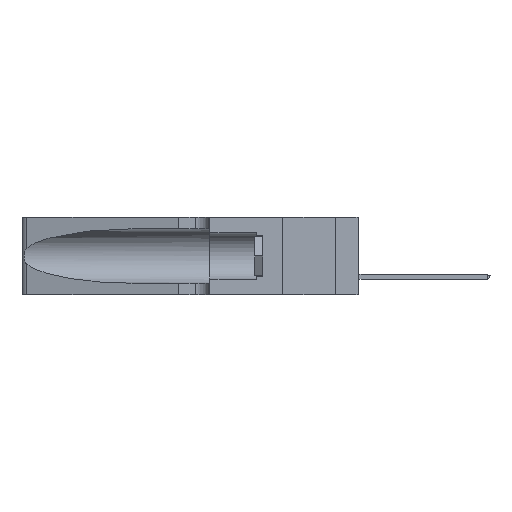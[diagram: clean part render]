
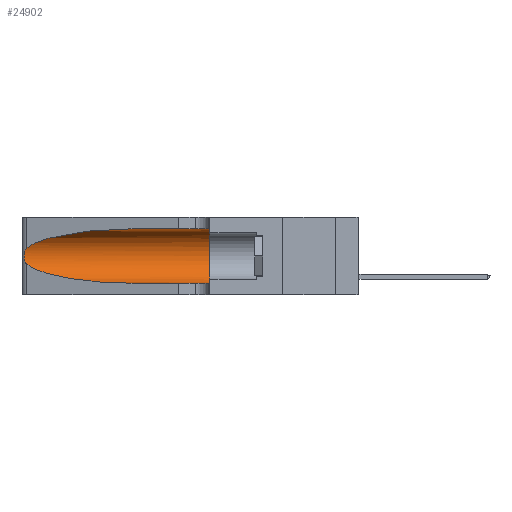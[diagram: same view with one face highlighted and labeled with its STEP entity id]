
A CAD part, left-side view. The second image highlights one B-rep face of the part: STEP entity #24902.
In plain terms, the highlighted cylindrical face has radius 3.308 mm (diameter 6.617 mm), a partial arc.
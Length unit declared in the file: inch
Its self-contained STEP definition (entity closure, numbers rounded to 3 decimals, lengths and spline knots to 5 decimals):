
#1590 = CARTESIAN_POINT ( 'NONE',  ( 0.1305, 0.35, 0.31525 ) ) ;
#2297 = CYLINDRICAL_SURFACE ( 'NONE', #27522, 0.13025 ) ;
#3438 = FACE_OUTER_BOUND ( 'NONE', #16273, .T. ) ;
#4509 = CARTESIAN_POINT ( 'NONE',  ( 0.25487, 1.22718, 0.14631 ) ) ;
#4609 = EDGE_CURVE ( 'NONE', #43980, #24915, #43379, .T. ) ;
#4656 = LINE ( 'NONE', #34526, #8044 ) ;
#4694 = AXIS2_PLACEMENT_3D ( 'NONE', #8359, #11439, #29441 ) ;
#4831 = CARTESIAN_POINT ( 'NONE',  ( 0.18966, 0.96281, 0.05475 ) ) ;
#5247 = CARTESIAN_POINT ( 'NONE',  ( 0.25487, 1.22718, 0.14631 ) ) ;
#6354 = VERTEX_POINT ( 'NONE', #29398 ) ;
#7000 = DIRECTION ( 'NONE',  ( 0., 0., -1. ) ) ;
#7172 = CIRCLE ( 'NONE', #4694, 0.13025 ) ;
#7334 = CARTESIAN_POINT ( 'NONE',  ( 0.25555, 1.22994, 0.2215 ) ) ;
#8044 = VECTOR ( 'NONE', #31187, 39.37008 ) ;
#8359 = CARTESIAN_POINT ( 'NONE',  ( 0.1305, 0.35, 0.185 ) ) ;
#8388 = CARTESIAN_POINT ( 'NONE',  ( 0.26075, 1.23896, 0.178 ) ) ;
#9094 = DIRECTION ( 'NONE',  ( 0., -1., 0. ) ) ;
#9400 = LINE ( 'NONE', #22945, #34593 ) ;
#10596 = VERTEX_POINT ( 'NONE', #11961 ) ;
#10973 = ORIENTED_EDGE ( 'NONE', *, *, #45958, .T. ) ;
#10992 = CARTESIAN_POINT ( 'NONE',  ( 0.25487, 1.22718, 0.22369 ) ) ;
#11439 = DIRECTION ( 'NONE',  ( 0., 1., 0. ) ) ;
#11451 = CARTESIAN_POINT ( 'NONE',  ( 0.1305, 0.72297, 0.31525 ) ) ;
#11626 = CARTESIAN_POINT ( 'NONE',  ( 0.26017, 1.23833, 0.17102 ) ) ;
#11686 = CARTESIAN_POINT ( 'NONE',  ( 0.1305, 0.72297, 0.05475 ) ) ;
#11929 = ORIENTED_EDGE ( 'NONE', *, *, #16761, .T. ) ;
#11961 = CARTESIAN_POINT ( 'NONE',  ( 0.1305, 0.35, 0.05475 ) ) ;
#13103 = EDGE_CURVE ( 'NONE', #18558, #10596, #7172, .T. ) ;
#13581 = EDGE_CURVE ( 'NONE', #6354, #10596, #9400, .T. ) ;
#14682 = B_SPLINE_CURVE_WITH_KNOTS ( 'NONE', 3,
 ( #17909, #7334, #32454, #32601, #36290, #26000, #36901, #8388, #11626, #30110, #37053, #44227, #40180, #18646 ),
 .UNSPECIFIED., .F., .F.,
 ( 4, 2, 2, 2, 2, 2, 4 ),
 ( 0., 0.00027, 0.00053, 0.00107, 0.0016, 0.00187, 0.00214 ),
 .UNSPECIFIED. ) ;
#16273 = EDGE_LOOP ( 'NONE', ( #33020, #11929, #10973, #35952, #36007, #21637 ) ) ;
#16761 = EDGE_CURVE ( 'NONE', #24915, #22778, #14682, .T. ) ;
#16793 = CARTESIAN_POINT ( 'NONE',  ( 0.2373, 1.15595, 0.28018 ) ) ;
#17909 = CARTESIAN_POINT ( 'NONE',  ( 0.25487, 1.22718, 0.22369 ) ) ;
#17931 = CARTESIAN_POINT ( 'NONE',  ( 0.1305, 1.61858, 0.185 ) ) ;
#18558 = VERTEX_POINT ( 'NONE', #1590 ) ;
#18646 = CARTESIAN_POINT ( 'NONE',  ( 0.25487, 1.22718, 0.14631 ) ) ;
#21637 = ORIENTED_EDGE ( 'NONE', *, *, #26189, .F. ) ;
#22778 = VERTEX_POINT ( 'NONE', #5247 ) ;
#22945 = CARTESIAN_POINT ( 'NONE',  ( 0.1305, 1.61858, 0.05475 ) ) ;
#23805 = CARTESIAN_POINT ( 'NONE',  ( 0.1305, 0.72297, 0.31525 ) ) ;
#24902 = ADVANCED_FACE ( 'NONE', ( #3438 ), #2297, .F. ) ;
#24915 = VERTEX_POINT ( 'NONE', #10992 ) ;
#26000 = CARTESIAN_POINT ( 'NONE',  ( 0.26018, 1.23835, 0.19895 ) ) ;
#26189 = EDGE_CURVE ( 'NONE', #43980, #18558, #4656, .T. ) ;
#27522 = AXIS2_PLACEMENT_3D ( 'NONE', #17931, #38979, #7000 ) ;
#28202 = CARTESIAN_POINT ( 'NONE',  ( 0.25487, 1.22718, 0.22369 ) ) ;
#29398 = CARTESIAN_POINT ( 'NONE',  ( 0.1305, 0.72297, 0.05475 ) ) ;
#29441 = DIRECTION ( 'NONE',  ( 0., 0., 1. ) ) ;
#30110 = CARTESIAN_POINT ( 'NONE',  ( 0.25856, 1.23593, 0.16098 ) ) ;
#31187 = DIRECTION ( 'NONE',  ( 0., -1., 0. ) ) ;
#32454 = CARTESIAN_POINT ( 'NONE',  ( 0.25639, 1.23184, 0.21858 ) ) ;
#32601 = CARTESIAN_POINT ( 'NONE',  ( 0.25787, 1.23484, 0.2124 ) ) ;
#33020 = ORIENTED_EDGE ( 'NONE', *, *, #4609, .T. ) ;
#34219 =( BOUNDED_CURVE ( )  B_SPLINE_CURVE ( 3, ( #4509, #36650, #4831, #11686 ),
 .UNSPECIFIED., .F., .T. ) 
 B_SPLINE_CURVE_WITH_KNOTS ( ( 4, 4 ),
 ( 3.44316, 4.71239 ),
 .UNSPECIFIED. ) 
 CURVE ( )  GEOMETRIC_REPRESENTATION_ITEM ( )  RATIONAL_B_SPLINE_CURVE ( ( 1., 0.87, 0.87, 1. ) ) 
 REPRESENTATION_ITEM ( '' )  );
#34526 = CARTESIAN_POINT ( 'NONE',  ( 0.1305, 1.61858, 0.31525 ) ) ;
#34593 = VECTOR ( 'NONE', #9094, 39.37008 ) ;
#35952 = ORIENTED_EDGE ( 'NONE', *, *, #13581, .T. ) ;
#36007 = ORIENTED_EDGE ( 'NONE', *, *, #13103, .F. ) ;
#36290 = CARTESIAN_POINT ( 'NONE',  ( 0.25854, 1.2359, 0.20912 ) ) ;
#36650 = CARTESIAN_POINT ( 'NONE',  ( 0.2373, 1.15595, 0.08982 ) ) ;
#36901 = CARTESIAN_POINT ( 'NONE',  ( 0.26075, 1.23896, 0.19203 ) ) ;
#37053 = CARTESIAN_POINT ( 'NONE',  ( 0.25789, 1.23486, 0.15765 ) ) ;
#38979 = DIRECTION ( 'NONE',  ( 0., -1., 0. ) ) ;
#40180 = CARTESIAN_POINT ( 'NONE',  ( 0.25555, 1.22993, 0.14849 ) ) ;
#40800 = CARTESIAN_POINT ( 'NONE',  ( 0.18966, 0.96281, 0.31525 ) ) ;
#43379 =( BOUNDED_CURVE ( )  B_SPLINE_CURVE ( 3, ( #11451, #40800, #16793, #28202 ),
 .UNSPECIFIED., .F., .F. ) 
 B_SPLINE_CURVE_WITH_KNOTS ( ( 4, 4 ),
 ( 1.5708, 2.84003 ),
 .UNSPECIFIED. ) 
 CURVE ( )  GEOMETRIC_REPRESENTATION_ITEM ( )  RATIONAL_B_SPLINE_CURVE ( ( 1., 0.87, 0.87, 1. ) ) 
 REPRESENTATION_ITEM ( '' )  );
#43980 = VERTEX_POINT ( 'NONE', #23805 ) ;
#44227 = CARTESIAN_POINT ( 'NONE',  ( 0.25639, 1.23186, 0.15144 ) ) ;
#45958 = EDGE_CURVE ( 'NONE', #22778, #6354, #34219, .T. ) ;
